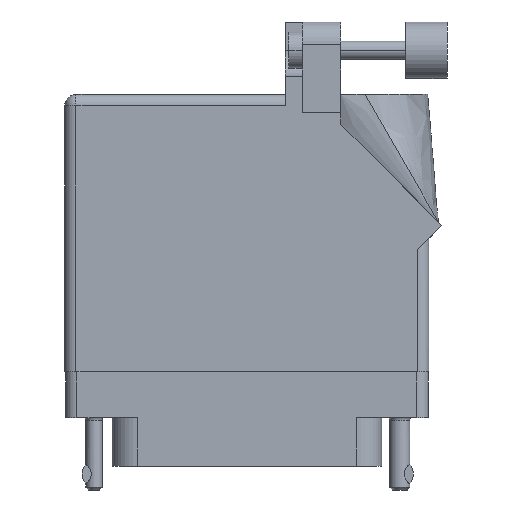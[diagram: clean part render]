
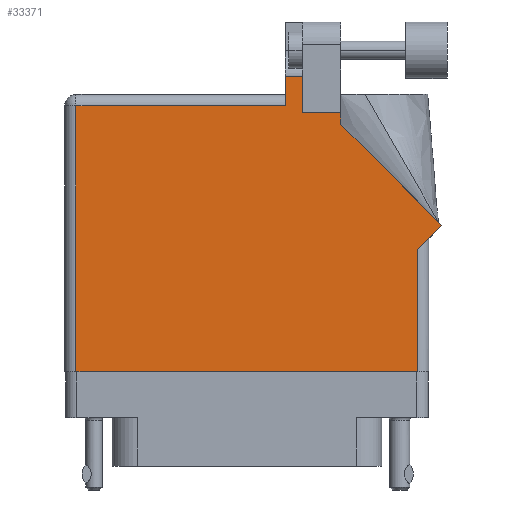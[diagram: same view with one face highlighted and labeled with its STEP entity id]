
A CAD part, front view. The second image highlights one B-rep face of the part: STEP entity #33371.
In plain terms, the highlighted face is planar.
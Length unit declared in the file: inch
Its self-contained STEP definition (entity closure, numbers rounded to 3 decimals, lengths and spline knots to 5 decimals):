
#2195 = DIRECTION ( 'NONE',  ( 0., -1., 0. ) ) ;
#2432 = VERTEX_POINT ( 'NONE', #39698 ) ;
#3602 = LINE ( 'NONE', #17545, #45608 ) ;
#3929 = CARTESIAN_POINT ( 'NONE',  ( 0.212, 1.368, 0.455 ) ) ;
#4459 = CARTESIAN_POINT ( 'NONE',  ( 0.943, -0.1, 0.455 ) ) ;
#4506 = EDGE_CURVE ( 'NONE', #10462, #45088, #20411, .T. ) ;
#4551 = DIRECTION ( 'NONE',  ( -1., 0., 0. ) ) ;
#4666 = VECTOR ( 'NONE', #2195, 39.37008 ) ;
#4992 = EDGE_CURVE ( 'NONE', #26359, #10462, #35415, .T. ) ;
#5026 = ORIENTED_EDGE ( 'NONE', *, *, #7243, .T. ) ;
#5050 = CARTESIAN_POINT ( 'NONE',  ( 0.943, 0.637, 0.455 ) ) ;
#5154 = AXIS2_PLACEMENT_3D ( 'NONE', #17185, #21440, #9601 ) ;
#6536 = VERTEX_POINT ( 'NONE', #14792 ) ;
#6822 = ORIENTED_EDGE ( 'NONE', *, *, #33055, .T. ) ;
#6986 = DIRECTION ( 'NONE',  ( 0.707, 0.707, 0. ) ) ;
#7243 = EDGE_CURVE ( 'NONE', #6536, #45695, #41216, .T. ) ;
#7860 = VERTEX_POINT ( 'NONE', #11664 ) ;
#8324 = VECTOR ( 'NONE', #4551, 39.37008 ) ;
#9601 = DIRECTION ( 'NONE',  ( -1., 0., 0. ) ) ;
#9667 = CARTESIAN_POINT ( 'NONE',  ( -0.943, -0.1, 0.455 ) ) ;
#10462 = VERTEX_POINT ( 'NONE', #30687 ) ;
#11159 = VECTOR ( 'NONE', #30742, 39.37008 ) ;
#11630 = DIRECTION ( 'NONE',  ( -1., 0., 0. ) ) ;
#11664 = CARTESIAN_POINT ( 'NONE',  ( 1.07571, 0.70771, 0.455 ) ) ;
#12183 = CARTESIAN_POINT ( 'NONE',  ( 0.212, 1.5315, 0.455 ) ) ;
#13463 = ORIENTED_EDGE ( 'NONE', *, *, #23785, .T. ) ;
#14604 = VECTOR ( 'NONE', #11630, 39.37008 ) ;
#14792 = CARTESIAN_POINT ( 'NONE',  ( -0.943, -0.1, 0.455 ) ) ;
#14879 = ORIENTED_EDGE ( 'NONE', *, *, #45087, .T. ) ;
#16599 = LINE ( 'NONE', #9667, #4666 ) ;
#16951 = ORIENTED_EDGE ( 'NONE', *, *, #42721, .T. ) ;
#17185 = CARTESIAN_POINT ( 'NONE',  ( -1.005, 1.43, 0.455 ) ) ;
#17545 = CARTESIAN_POINT ( 'NONE',  ( 1.005, 0.637, 0.455 ) ) ;
#18386 = DIRECTION ( 'NONE',  ( 0., 1., 0. ) ) ;
#18542 = CARTESIAN_POINT ( 'NONE',  ( -0.943, 1.368, 0.455 ) ) ;
#20150 = EDGE_CURVE ( 'NONE', #45695, #2432, #29580, .T. ) ;
#20411 = LINE ( 'NONE', #35136, #8324 ) ;
#21440 = DIRECTION ( 'NONE',  ( 0., 0., -1. ) ) ;
#21566 = CARTESIAN_POINT ( 'NONE',  ( 0.519, 1.26442, 0.455 ) ) ;
#23785 = EDGE_CURVE ( 'NONE', #7860, #26359, #34084, .T. ) ;
#24926 = EDGE_CURVE ( 'NONE', #33746, #41919, #45378, .T. ) ;
#26359 = VERTEX_POINT ( 'NONE', #21566 ) ;
#27019 = EDGE_CURVE ( 'NONE', #43102, #6536, #16599, .T. ) ;
#27190 = DIRECTION ( 'NONE',  ( -1., 0., 0. ) ) ;
#29580 = LINE ( 'NONE', #5050, #37408 ) ;
#29983 = CARTESIAN_POINT ( 'NONE',  ( 0.519, 1.26442, 0.455 ) ) ;
#30246 = CARTESIAN_POINT ( 'NONE',  ( 0.306, 1.33, 0.455 ) ) ;
#30687 = CARTESIAN_POINT ( 'NONE',  ( 0.519, 1.33, 0.455 ) ) ;
#30742 = DIRECTION ( 'NONE',  ( 1., 0., 0. ) ) ;
#31209 = CARTESIAN_POINT ( 'NONE',  ( -1.005, 1.368, 0.455 ) ) ;
#31824 = PLANE ( 'NONE',  #5154 ) ;
#32227 = DIRECTION ( 'NONE',  ( 0., 1., 0. ) ) ;
#33055 = EDGE_CURVE ( 'NONE', #2432, #7860, #3602, .T. ) ;
#33286 = CARTESIAN_POINT ( 'NONE',  ( 1.07571, 0.70771, 0.455 ) ) ;
#33368 = VECTOR ( 'NONE', #34805, 39.37008 ) ;
#33371 = ADVANCED_FACE ( 'NONE', ( #37844 ), #31824, .F. ) ;
#33618 = CARTESIAN_POINT ( 'NONE',  ( 0.212, 1.43, 0.455 ) ) ;
#33746 = VERTEX_POINT ( 'NONE', #12183 ) ;
#33891 = ORIENTED_EDGE ( 'NONE', *, *, #4992, .T. ) ;
#34084 = LINE ( 'NONE', #33286, #37705 ) ;
#34527 = CARTESIAN_POINT ( 'NONE',  ( 0.63677, 1.5315, 0.455 ) ) ;
#34805 = DIRECTION ( 'NONE',  ( 0., -1., 0. ) ) ;
#35136 = CARTESIAN_POINT ( 'NONE',  ( 0.519, 1.33, 0.455 ) ) ;
#35415 = LINE ( 'NONE', #29983, #48506 ) ;
#36301 = LINE ( 'NONE', #34527, #14604 ) ;
#36865 = ORIENTED_EDGE ( 'NONE', *, *, #24926, .T. ) ;
#37408 = VECTOR ( 'NONE', #32227, 39.37008 ) ;
#37705 = VECTOR ( 'NONE', #40518, 39.37008 ) ;
#37844 = FACE_OUTER_BOUND ( 'NONE', #41475, .T. ) ;
#38217 = LINE ( 'NONE', #31209, #44206 ) ;
#39698 = CARTESIAN_POINT ( 'NONE',  ( 0.943, 0.575, 0.455 ) ) ;
#40518 = DIRECTION ( 'NONE',  ( -0.707, 0.707, 0. ) ) ;
#41216 = LINE ( 'NONE', #45519, #11159 ) ;
#41475 = EDGE_LOOP ( 'NONE', ( #48566, #14879, #36865, #16951, #43276, #5026, #46423, #6822, #13463, #33891, #49037 ) ) ;
#41919 = VERTEX_POINT ( 'NONE', #3929 ) ;
#42721 = EDGE_CURVE ( 'NONE', #41919, #43102, #38217, .T. ) ;
#42916 = CARTESIAN_POINT ( 'NONE',  ( 0.306, 1.33, 0.455 ) ) ;
#43102 = VERTEX_POINT ( 'NONE', #18542 ) ;
#43276 = ORIENTED_EDGE ( 'NONE', *, *, #27019, .T. ) ;
#44206 = VECTOR ( 'NONE', #27190, 39.37008 ) ;
#45007 = DIRECTION ( 'NONE',  ( 0., 1., 0. ) ) ;
#45087 = EDGE_CURVE ( 'NONE', #46478, #33746, #36301, .T. ) ;
#45088 = VERTEX_POINT ( 'NONE', #42916 ) ;
#45378 = LINE ( 'NONE', #33618, #33368 ) ;
#45519 = CARTESIAN_POINT ( 'NONE',  ( -1.005, -0.1, 0.455 ) ) ;
#45601 = VECTOR ( 'NONE', #45007, 39.37008 ) ;
#45608 = VECTOR ( 'NONE', #6986, 39.37008 ) ;
#45695 = VERTEX_POINT ( 'NONE', #4459 ) ;
#46423 = ORIENTED_EDGE ( 'NONE', *, *, #20150, .T. ) ;
#46478 = VERTEX_POINT ( 'NONE', #49224 ) ;
#47761 = EDGE_CURVE ( 'NONE', #45088, #46478, #47974, .T. ) ;
#47974 = LINE ( 'NONE', #30246, #45601 ) ;
#48506 = VECTOR ( 'NONE', #18386, 39.37008 ) ;
#48566 = ORIENTED_EDGE ( 'NONE', *, *, #47761, .T. ) ;
#49037 = ORIENTED_EDGE ( 'NONE', *, *, #4506, .T. ) ;
#49224 = CARTESIAN_POINT ( 'NONE',  ( 0.306, 1.5315, 0.455 ) ) ;
